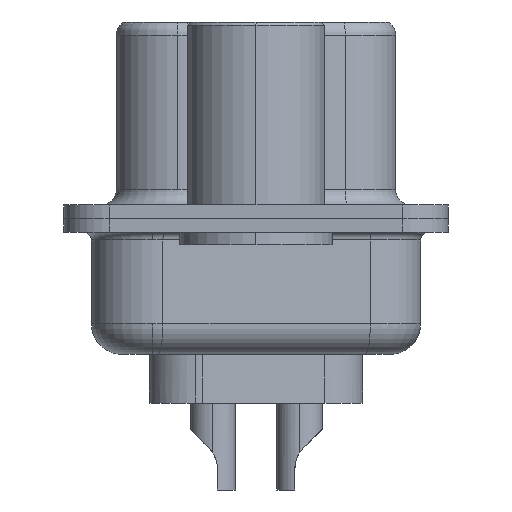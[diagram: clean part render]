
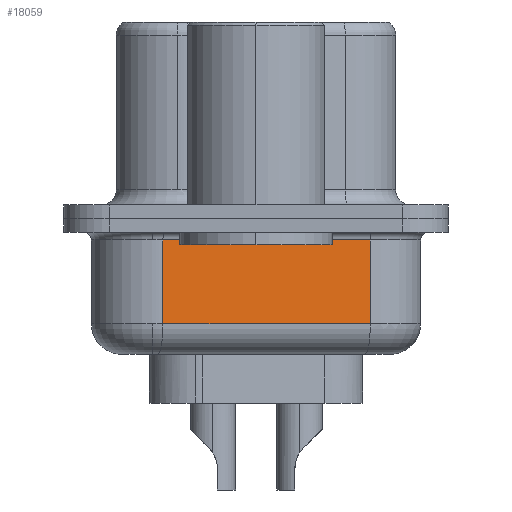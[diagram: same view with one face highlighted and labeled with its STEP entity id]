
A CAD part, left-side view. The second image highlights one B-rep face of the part: STEP entity #18059.
In plain terms, the highlighted planar face has unit normal (-0.985, -0.174, 0).
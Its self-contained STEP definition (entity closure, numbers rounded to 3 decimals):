
#199 = ORIENTED_EDGE ( 'NONE', *, *, #6927, .T. ) ;
#1172 = VECTOR ( 'NONE', #16075, 1000. ) ;
#2691 = VECTOR ( 'NONE', #12412, 1000. ) ;
#3282 = DIRECTION ( 'NONE',  ( -0.174, 0.985, 0. ) ) ;
#3339 = DIRECTION ( 'NONE',  ( 0., 0., 1. ) ) ;
#4027 = ORIENTED_EDGE ( 'NONE', *, *, #15699, .F. ) ;
#5071 = CARTESIAN_POINT ( 'NONE',  ( 2.85, 3.053, -4.45 ) ) ;
#5112 = LINE ( 'NONE', #23168, #2691 ) ;
#5621 = CARTESIAN_POINT ( 'NONE',  ( 4.049, -3.747, -0.7 ) ) ;
#5748 = EDGE_CURVE ( 'NONE', #22304, #17227, #8945, .T. ) ;
#6137 = CARTESIAN_POINT ( 'NONE',  ( 2.85, 3.053, -0.7 ) ) ;
#6806 = DIRECTION ( 'NONE',  ( -0.174, 0.985, 0. ) ) ;
#6927 = EDGE_CURVE ( 'NONE', #17227, #15260, #23069, .T. ) ;
#7448 = VERTEX_POINT ( 'NONE', #17467 ) ;
#8353 = CARTESIAN_POINT ( 'NONE',  ( 2.85, 3.053, -0.7 ) ) ;
#8945 = LINE ( 'NONE', #17855, #1172 ) ;
#9245 = ORIENTED_EDGE ( 'NONE', *, *, #5748, .T. ) ;
#9381 = VECTOR ( 'NONE', #6806, 1000. ) ;
#9890 = LINE ( 'NONE', #22574, #19660 ) ;
#10282 = AXIS2_PLACEMENT_3D ( 'NONE', #5071, #19558, #3282 ) ;
#11186 = CARTESIAN_POINT ( 'NONE',  ( 4.049, -3.747, -3.45 ) ) ;
#12412 = DIRECTION ( 'NONE',  ( 0.174, -0.985, 0. ) ) ;
#13560 = EDGE_LOOP ( 'NONE', ( #4027, #22287, #9245, #199 ) ) ;
#14108 = PLANE ( 'NONE',  #10282 ) ;
#15260 = VERTEX_POINT ( 'NONE', #6137 ) ;
#15699 = EDGE_CURVE ( 'NONE', #7448, #15260, #9890, .T. ) ;
#16075 = DIRECTION ( 'NONE',  ( 0., 0., 1. ) ) ;
#17227 = VERTEX_POINT ( 'NONE', #5621 ) ;
#17467 = CARTESIAN_POINT ( 'NONE',  ( 2.85, 3.053, -3.45 ) ) ;
#17855 = CARTESIAN_POINT ( 'NONE',  ( 4.049, -3.747, -4.45 ) ) ;
#18059 = ADVANCED_FACE ( 'NONE', ( #23128 ), #14108, .F. ) ;
#19041 = EDGE_CURVE ( 'NONE', #7448, #22304, #5112, .T. ) ;
#19558 = DIRECTION ( 'NONE',  ( 0.985, 0.174, 0. ) ) ;
#19660 = VECTOR ( 'NONE', #3339, 1000. ) ;
#22287 = ORIENTED_EDGE ( 'NONE', *, *, #19041, .T. ) ;
#22304 = VERTEX_POINT ( 'NONE', #11186 ) ;
#22574 = CARTESIAN_POINT ( 'NONE',  ( 2.85, 3.053, -4.45 ) ) ;
#23069 = LINE ( 'NONE', #8353, #9381 ) ;
#23128 = FACE_OUTER_BOUND ( 'NONE', #13560, .T. ) ;
#23168 = CARTESIAN_POINT ( 'NONE',  ( 2.85, 3.053, -3.45 ) ) ;
